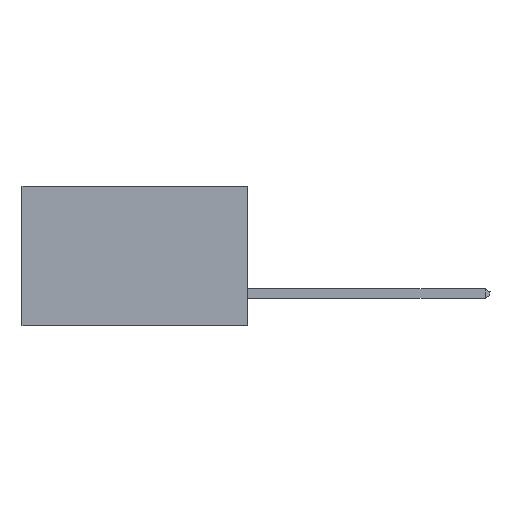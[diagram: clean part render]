
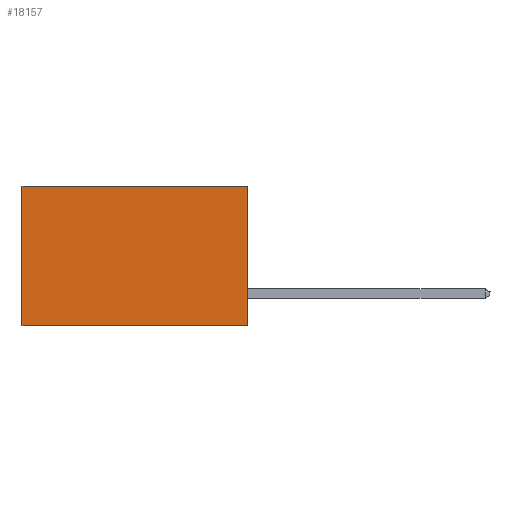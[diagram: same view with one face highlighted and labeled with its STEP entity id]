
A CAD part, left-side view. The second image highlights one B-rep face of the part: STEP entity #18157.
In plain terms, the highlighted planar face has unit normal (-1, 0, 0).
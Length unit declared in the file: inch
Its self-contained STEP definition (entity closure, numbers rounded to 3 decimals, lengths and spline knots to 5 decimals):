
#583 = VECTOR ( 'NONE', #827, 39.37008 ) ;
#827 = DIRECTION ( 'NONE',  ( 0., 0., -1. ) ) ;
#1664 = DIRECTION ( 'NONE',  ( 0., 0., -1. ) ) ;
#1797 = CARTESIAN_POINT ( 'NONE',  ( 0.2615, 0.6, -0.37 ) ) ;
#2218 = EDGE_CURVE ( 'NONE', #22566, #12183, #8404, .T. ) ;
#2894 = CARTESIAN_POINT ( 'NONE',  ( 0.2615, 0., -0.37 ) ) ;
#3694 = CARTESIAN_POINT ( 'NONE',  ( 0.2615, 0., 0. ) ) ;
#4414 = AXIS2_PLACEMENT_3D ( 'NONE', #23912, #8706, #12921 ) ;
#4521 = EDGE_CURVE ( 'NONE', #22566, #12535, #14176, .T. ) ;
#4660 = ORIENTED_EDGE ( 'NONE', *, *, #15885, .F. ) ;
#5409 = LINE ( 'NONE', #1797, #11941 ) ;
#5546 = ORIENTED_EDGE ( 'NONE', *, *, #8195, .T. ) ;
#5782 = VECTOR ( 'NONE', #21437, 39.37008 ) ;
#6868 = LINE ( 'NONE', #2894, #8488 ) ;
#8195 = EDGE_CURVE ( 'NONE', #12535, #18204, #5409, .T. ) ;
#8404 = LINE ( 'NONE', #17916, #583 ) ;
#8488 = VECTOR ( 'NONE', #10470, 39.37008 ) ;
#8706 = DIRECTION ( 'NONE',  ( 1., 0., 0. ) ) ;
#9477 = ORIENTED_EDGE ( 'NONE', *, *, #2218, .F. ) ;
#9940 = CARTESIAN_POINT ( 'NONE',  ( 0.2615, 0., 0. ) ) ;
#10470 = DIRECTION ( 'NONE',  ( 0., 1., 0. ) ) ;
#10572 = PLANE ( 'NONE',  #4414 ) ;
#11941 = VECTOR ( 'NONE', #1664, 39.37008 ) ;
#12183 = VERTEX_POINT ( 'NONE', #18229 ) ;
#12535 = VERTEX_POINT ( 'NONE', #19318 ) ;
#12921 = DIRECTION ( 'NONE',  ( 0., 0., -1. ) ) ;
#14176 = LINE ( 'NONE', #9940, #5782 ) ;
#15885 = EDGE_CURVE ( 'NONE', #12183, #18204, #6868, .T. ) ;
#17916 = CARTESIAN_POINT ( 'NONE',  ( 0.2615, 0., -0.37 ) ) ;
#18157 = ADVANCED_FACE ( 'NONE', ( #22419 ), #10572, .F. ) ;
#18204 = VERTEX_POINT ( 'NONE', #18933 ) ;
#18229 = CARTESIAN_POINT ( 'NONE',  ( 0.2615, 0., -0.37 ) ) ;
#18933 = CARTESIAN_POINT ( 'NONE',  ( 0.2615, 0.6, -0.37 ) ) ;
#19318 = CARTESIAN_POINT ( 'NONE',  ( 0.2615, 0.6, 0. ) ) ;
#19465 = EDGE_LOOP ( 'NONE', ( #5546, #4660, #9477, #21824 ) ) ;
#21437 = DIRECTION ( 'NONE',  ( 0., 1., 0. ) ) ;
#21824 = ORIENTED_EDGE ( 'NONE', *, *, #4521, .T. ) ;
#22419 = FACE_OUTER_BOUND ( 'NONE', #19465, .T. ) ;
#22566 = VERTEX_POINT ( 'NONE', #3694 ) ;
#23912 = CARTESIAN_POINT ( 'NONE',  ( 0.2615, 0., -0.37 ) ) ;
